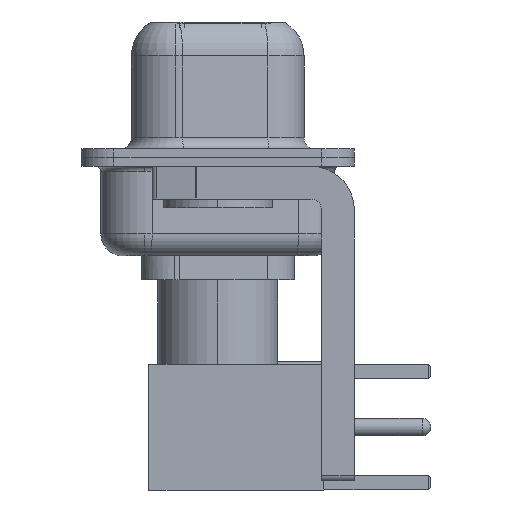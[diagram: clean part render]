
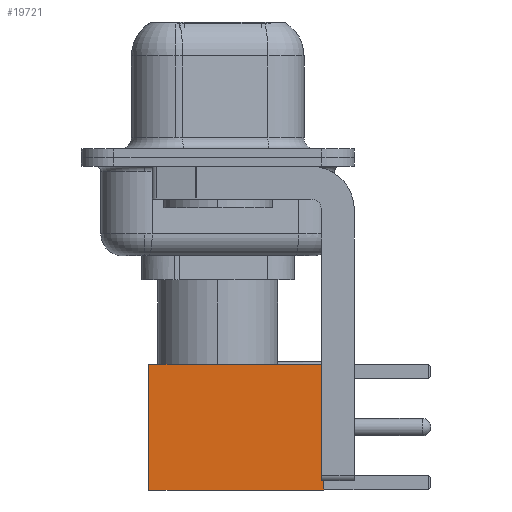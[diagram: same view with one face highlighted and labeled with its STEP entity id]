
A CAD part, left-side view. The second image highlights one B-rep face of the part: STEP entity #19721.
In plain terms, the highlighted face is planar.
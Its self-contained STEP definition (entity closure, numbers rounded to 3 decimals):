
#1283 = CARTESIAN_POINT ( 'NONE',  ( 0., 2.875, 8. ) ) ;
#1373 = DIRECTION ( 'NONE',  ( 0., 0., 1. ) ) ;
#2041 = CARTESIAN_POINT ( 'NONE',  ( 2.875, 2.875, 0. ) ) ;
#2364 = CARTESIAN_POINT ( 'NONE',  ( -2.875, 2.875, 8. ) ) ;
#3389 = ORIENTED_EDGE ( 'NONE', *, *, #7784, .T. ) ;
#3764 = LINE ( 'NONE', #12748, #22845 ) ;
#4185 = VECTOR ( 'NONE', #8412, 1000. ) ;
#4921 = VERTEX_POINT ( 'NONE', #2364 ) ;
#5372 = DIRECTION ( 'NONE',  ( 0., 0., -1. ) ) ;
#5950 = EDGE_CURVE ( 'NONE', #6576, #20170, #20221, .T. ) ;
#6576 = VERTEX_POINT ( 'NONE', #25341 ) ;
#7784 = EDGE_CURVE ( 'NONE', #20170, #21023, #3764, .T. ) ;
#8412 = DIRECTION ( 'NONE',  ( -1., 0., 0. ) ) ;
#10082 = PLANE ( 'NONE',  #13220 ) ;
#10235 = EDGE_CURVE ( 'NONE', #6576, #4921, #20972, .T. ) ;
#10710 = ORIENTED_EDGE ( 'NONE', *, *, #5950, .T. ) ;
#11514 = CARTESIAN_POINT ( 'NONE',  ( -2.875, 2.875, 0. ) ) ;
#12479 = DIRECTION ( 'NONE',  ( -1., 0., 0. ) ) ;
#12748 = CARTESIAN_POINT ( 'NONE',  ( 0., 2.875, 0. ) ) ;
#12862 = EDGE_LOOP ( 'NONE', ( #10710, #3389, #16890, #27747 ) ) ;
#13220 = AXIS2_PLACEMENT_3D ( 'NONE', #16761, #25651, #1373 ) ;
#13508 = LINE ( 'NONE', #11514, #17245 ) ;
#13521 = CARTESIAN_POINT ( 'NONE',  ( 2.875, 2.875, 0. ) ) ;
#16761 = CARTESIAN_POINT ( 'NONE',  ( 2.875, 2.875, 0. ) ) ;
#16890 = ORIENTED_EDGE ( 'NONE', *, *, #18061, .F. ) ;
#17245 = VECTOR ( 'NONE', #24376, 1000. ) ;
#18061 = EDGE_CURVE ( 'NONE', #4921, #21023, #13508, .T. ) ;
#19721 = ADVANCED_FACE ( 'NONE', ( #25502 ), #10082, .T. ) ;
#20170 = VERTEX_POINT ( 'NONE', #2041 ) ;
#20221 = LINE ( 'NONE', #13521, #24555 ) ;
#20972 = LINE ( 'NONE', #1283, #4185 ) ;
#21023 = VERTEX_POINT ( 'NONE', #22596 ) ;
#22596 = CARTESIAN_POINT ( 'NONE',  ( -2.875, 2.875, 0. ) ) ;
#22845 = VECTOR ( 'NONE', #12479, 1000. ) ;
#24376 = DIRECTION ( 'NONE',  ( 0., 0., -1. ) ) ;
#24555 = VECTOR ( 'NONE', #5372, 1000. ) ;
#25341 = CARTESIAN_POINT ( 'NONE',  ( 2.875, 2.875, 8. ) ) ;
#25502 = FACE_OUTER_BOUND ( 'NONE', #12862, .T. ) ;
#25651 = DIRECTION ( 'NONE',  ( 0., 1., 0. ) ) ;
#27747 = ORIENTED_EDGE ( 'NONE', *, *, #10235, .F. ) ;
